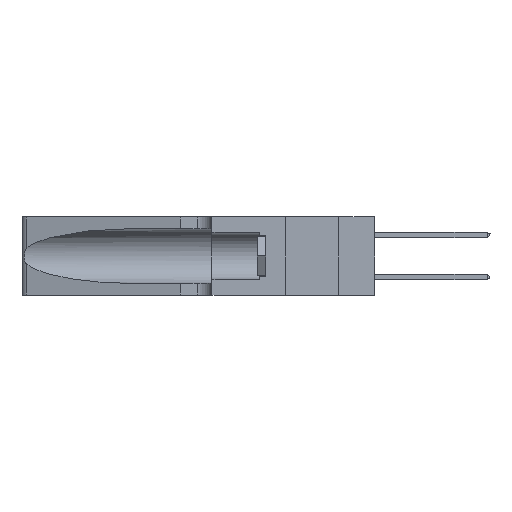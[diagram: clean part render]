
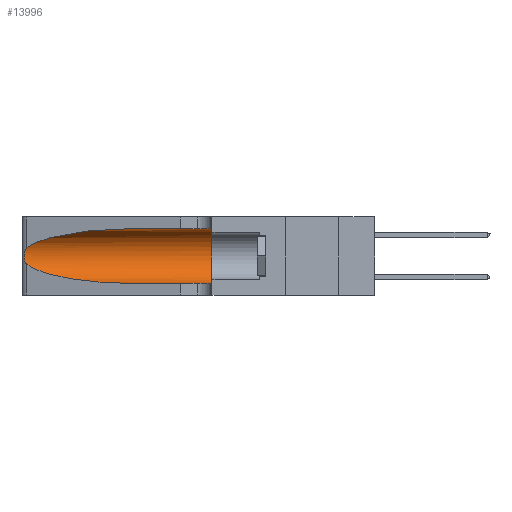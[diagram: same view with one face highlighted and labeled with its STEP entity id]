
A CAD part, left-side view. The second image highlights one B-rep face of the part: STEP entity #13996.
In plain terms, the highlighted cylindrical face has radius 3.308 mm (diameter 6.617 mm), a partial arc.
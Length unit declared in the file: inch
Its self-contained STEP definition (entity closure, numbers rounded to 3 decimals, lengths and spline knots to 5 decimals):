
#202 = ORIENTED_EDGE ( 'NONE', *, *, #12437, .F. ) ;
#2006 = CARTESIAN_POINT ( 'NONE',  ( 0.25555, 1.22994, 0.2215 ) ) ;
#2117 = VECTOR ( 'NONE', #25434, 39.37008 ) ;
#2630 = ORIENTED_EDGE ( 'NONE', *, *, #4069, .T. ) ;
#3369 = EDGE_CURVE ( 'NONE', #38462, #20594, #28840, .T. ) ;
#3459 = CARTESIAN_POINT ( 'NONE',  ( 0.18966, 0.96281, 0.05475 ) ) ;
#4069 = EDGE_CURVE ( 'NONE', #7554, #37561, #30656, .T. ) ;
#5200 = LINE ( 'NONE', #27452, #35547 ) ;
#5444 = CARTESIAN_POINT ( 'NONE',  ( 0.25555, 1.22993, 0.14849 ) ) ;
#6226 = CARTESIAN_POINT ( 'NONE',  ( 0.1305, 0.72297, 0.31525 ) ) ;
#6506 = CARTESIAN_POINT ( 'NONE',  ( 0.2373, 1.15595, 0.08982 ) ) ;
#7507 = CARTESIAN_POINT ( 'NONE',  ( 0.1305, 0.72297, 0.31525 ) ) ;
#7554 = VERTEX_POINT ( 'NONE', #7507 ) ;
#8314 = VERTEX_POINT ( 'NONE', #20762 ) ;
#8451 = DIRECTION ( 'NONE',  ( 0., -1., 0. ) ) ;
#8789 = DIRECTION ( 'NONE',  ( 0., -1., 0. ) ) ;
#8943 = CARTESIAN_POINT ( 'NONE',  ( 0.26017, 1.23833, 0.17102 ) ) ;
#9775 = ORIENTED_EDGE ( 'NONE', *, *, #30994, .T. ) ;
#11097 = LINE ( 'NONE', #22016, #2117 ) ;
#12104 = CARTESIAN_POINT ( 'NONE',  ( 0.26018, 1.23835, 0.19895 ) ) ;
#12374 = CARTESIAN_POINT ( 'NONE',  ( 0.25789, 1.23486, 0.15765 ) ) ;
#12437 = EDGE_CURVE ( 'NONE', #7554, #19450, #11097, .T. ) ;
#12815 = CARTESIAN_POINT ( 'NONE',  ( 0.25487, 1.22718, 0.22369 ) ) ;
#13261 = DIRECTION ( 'NONE',  ( 0., 0., -1. ) ) ;
#13980 = ORIENTED_EDGE ( 'NONE', *, *, #17915, .T. ) ;
#13996 = ADVANCED_FACE ( 'NONE', ( #36180 ), #15789, .F. ) ;
#14704 = EDGE_LOOP ( 'NONE', ( #2630, #13980, #19240, #9775, #30406, #202 ) ) ;
#14733 = CARTESIAN_POINT ( 'NONE',  ( 0.1305, 0.35, 0.31525 ) ) ;
#15456 = CARTESIAN_POINT ( 'NONE',  ( 0.25487, 1.22718, 0.14631 ) ) ;
#15684 = DIRECTION ( 'NONE',  ( 0., 1., 0. ) ) ;
#15789 = CYLINDRICAL_SURFACE ( 'NONE', #36926, 0.13025 ) ;
#17859 = CARTESIAN_POINT ( 'NONE',  ( 0.25487, 1.22718, 0.22369 ) ) ;
#17915 = EDGE_CURVE ( 'NONE', #37561, #38462, #35753, .T. ) ;
#18857 = DIRECTION ( 'NONE',  ( 0., 0., 1. ) ) ;
#19240 = ORIENTED_EDGE ( 'NONE', *, *, #3369, .T. ) ;
#19274 = CARTESIAN_POINT ( 'NONE',  ( 0.1305, 0.72297, 0.05475 ) ) ;
#19450 = VERTEX_POINT ( 'NONE', #14733 ) ;
#20594 = VERTEX_POINT ( 'NONE', #28616 ) ;
#20762 = CARTESIAN_POINT ( 'NONE',  ( 0.1305, 0.35, 0.05475 ) ) ;
#21260 = CIRCLE ( 'NONE', #33116, 0.13025 ) ;
#21416 = CARTESIAN_POINT ( 'NONE',  ( 0.26075, 1.23896, 0.178 ) ) ;
#22016 = CARTESIAN_POINT ( 'NONE',  ( 0.1305, 1.61858, 0.31525 ) ) ;
#22500 = CARTESIAN_POINT ( 'NONE',  ( 0.2373, 1.15595, 0.28018 ) ) ;
#23364 = CARTESIAN_POINT ( 'NONE',  ( 0.1305, 1.61858, 0.185 ) ) ;
#24451 = CARTESIAN_POINT ( 'NONE',  ( 0.25854, 1.2359, 0.20912 ) ) ;
#25434 = DIRECTION ( 'NONE',  ( 0., -1., 0. ) ) ;
#26102 = CARTESIAN_POINT ( 'NONE',  ( 0.18966, 0.96281, 0.31525 ) ) ;
#27225 = CARTESIAN_POINT ( 'NONE',  ( 0.25487, 1.22718, 0.22369 ) ) ;
#27452 = CARTESIAN_POINT ( 'NONE',  ( 0.1305, 1.61858, 0.05475 ) ) ;
#27652 = CARTESIAN_POINT ( 'NONE',  ( 0.25639, 1.23186, 0.15144 ) ) ;
#28616 = CARTESIAN_POINT ( 'NONE',  ( 0.1305, 0.72297, 0.05475 ) ) ;
#28840 =( BOUNDED_CURVE ( )  B_SPLINE_CURVE ( 3, ( #35165, #6506, #3459, #19274 ),
 .UNSPECIFIED., .F., .F. ) 
 B_SPLINE_CURVE_WITH_KNOTS ( ( 4, 4 ),
 ( 3.44316, 4.71239 ),
 .UNSPECIFIED. ) 
 CURVE ( )  GEOMETRIC_REPRESENTATION_ITEM ( )  RATIONAL_B_SPLINE_CURVE ( ( 1., 0.87, 0.87, 1. ) ) 
 REPRESENTATION_ITEM ( '' )  );
#29416 = EDGE_CURVE ( 'NONE', #19450, #8314, #21260, .T. ) ;
#30406 = ORIENTED_EDGE ( 'NONE', *, *, #29416, .F. ) ;
#30656 =( BOUNDED_CURVE ( )  B_SPLINE_CURVE ( 3, ( #6226, #26102, #22500, #17859 ),
 .UNSPECIFIED., .F., .F. ) 
 B_SPLINE_CURVE_WITH_KNOTS ( ( 4, 4 ),
 ( 1.5708, 2.84003 ),
 .UNSPECIFIED. ) 
 CURVE ( )  GEOMETRIC_REPRESENTATION_ITEM ( )  RATIONAL_B_SPLINE_CURVE ( ( 1., 0.87, 0.87, 1. ) ) 
 REPRESENTATION_ITEM ( '' )  );
#30865 = CARTESIAN_POINT ( 'NONE',  ( 0.25787, 1.23484, 0.2124 ) ) ;
#30994 = EDGE_CURVE ( 'NONE', #20594, #8314, #5200, .T. ) ;
#33116 = AXIS2_PLACEMENT_3D ( 'NONE', #37959, #15684, #18857 ) ;
#33826 = CARTESIAN_POINT ( 'NONE',  ( 0.25639, 1.23184, 0.21858 ) ) ;
#34349 = CARTESIAN_POINT ( 'NONE',  ( 0.25487, 1.22718, 0.14631 ) ) ;
#35165 = CARTESIAN_POINT ( 'NONE',  ( 0.25487, 1.22718, 0.14631 ) ) ;
#35547 = VECTOR ( 'NONE', #8451, 39.37008 ) ;
#35753 = B_SPLINE_CURVE_WITH_KNOTS ( 'NONE', 3,
 ( #27225, #2006, #33826, #30865, #24451, #12104, #40778, #21416, #8943, #40635, #12374, #27652, #5444, #15456 ),
 .UNSPECIFIED., .F., .F.,
 ( 4, 2, 2, 2, 2, 2, 4 ),
 ( 0., 0.00027, 0.00053, 0.00107, 0.0016, 0.00187, 0.00214 ),
 .UNSPECIFIED. ) ;
#36180 = FACE_OUTER_BOUND ( 'NONE', #14704, .T. ) ;
#36926 = AXIS2_PLACEMENT_3D ( 'NONE', #23364, #8789, #13261 ) ;
#37561 = VERTEX_POINT ( 'NONE', #12815 ) ;
#37959 = CARTESIAN_POINT ( 'NONE',  ( 0.1305, 0.35, 0.185 ) ) ;
#38462 = VERTEX_POINT ( 'NONE', #34349 ) ;
#40635 = CARTESIAN_POINT ( 'NONE',  ( 0.25856, 1.23593, 0.16098 ) ) ;
#40778 = CARTESIAN_POINT ( 'NONE',  ( 0.26075, 1.23896, 0.19203 ) ) ;
